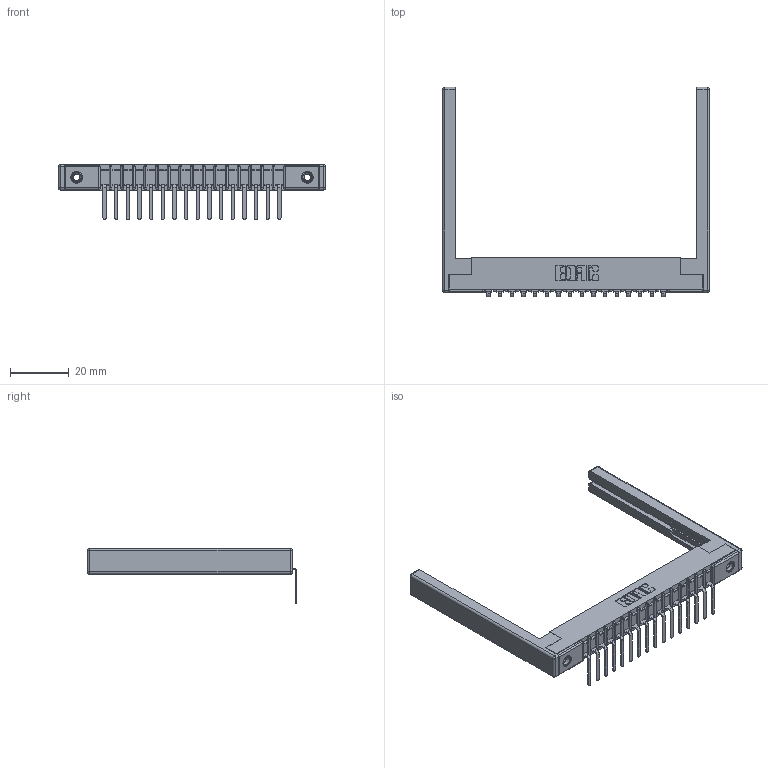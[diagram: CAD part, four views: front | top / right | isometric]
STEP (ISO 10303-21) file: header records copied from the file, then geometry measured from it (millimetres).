
FILE_DESCRIPTION (( 'STEP AP203' ), '1' );
FILE_NAME ('357-016-457-168.STEP', '2020-09-30T20:21:37', ( '' ), ( '' ), 'SwSTEP 2.0', 'SolidWorks 2020', '' );
FILE_SCHEMA (( 'CONFIG_CONTROL_DESIGN' ));
Length unit declared in the file: inch
Products named in the file (5): 357-016-457-168; 307-220-068; 345-250-001_345-250-001-102; 307-290-002_557; 307 Part_.156 Dia Mounting Holes
Assembly tree (21 placements, depth 2):
  357-016-457-168
    307 Part_.156 Dia Mounting Holes
    307-290-002_557  x16
    307-220-068  x2
    345-250-001_345-250-001-102  x2
Bounding box: 90.83 x 71.29 x 18.67 mm (x, y, z)
Volume: 10595.3 mm3; surface area: 14930.1 mm2
Topology: 21 solids, 21 shells, 1537 faces, 4617 edges, 3010 vertices
Faces by surface type: plane 910, cylinder 569, sphere 42, cone 12, torus 4
Entity records: 20535 total; most frequent: CARTESIAN_POINT 3425, ORIENTED_EDGE 3404, DIRECTION 3358, EDGE_CURVE 1702, VECTOR 1288, LINE 1288, VERTEX_POINT 1102, AXIS2_PLACEMENT_3D 1035
